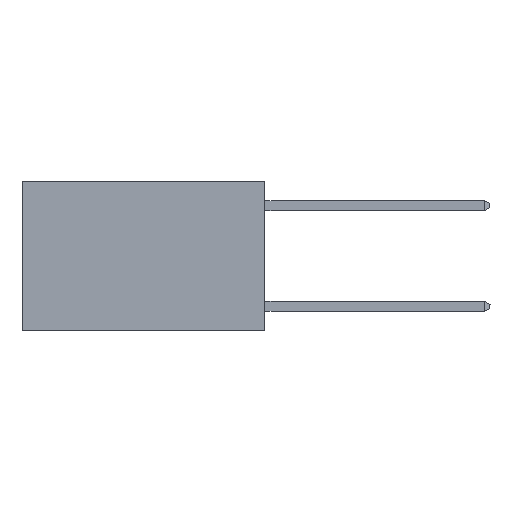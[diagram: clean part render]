
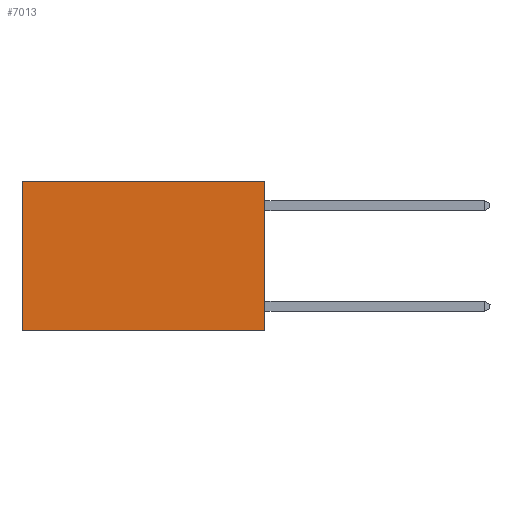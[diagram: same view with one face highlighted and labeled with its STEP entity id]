
A CAD part, left-side view. The second image highlights one B-rep face of the part: STEP entity #7013.
In plain terms, the highlighted planar face has unit normal (-1, 0, 0).
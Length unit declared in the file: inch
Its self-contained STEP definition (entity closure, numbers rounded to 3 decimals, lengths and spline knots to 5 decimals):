
#8 = ORIENTED_EDGE ( 'NONE', *, *, #19755, .T. ) ;
#76 = PLANE ( 'NONE',  #18630 ) ;
#163 = DIRECTION ( 'NONE',  ( 0., 0., -1. ) ) ;
#978 = VECTOR ( 'NONE', #23989, 39.37008 ) ;
#1407 = CARTESIAN_POINT ( 'NONE',  ( 0.2625, 0., -0.37 ) ) ;
#1803 = DIRECTION ( 'NONE',  ( 0., 1., 0. ) ) ;
#2769 = CARTESIAN_POINT ( 'NONE',  ( 0.2625, 0.6, 0. ) ) ;
#3751 = ORIENTED_EDGE ( 'NONE', *, *, #18861, .T. ) ;
#3913 = EDGE_CURVE ( 'NONE', #17899, #15839, #20355, .T. ) ;
#4371 = VERTEX_POINT ( 'NONE', #16931 ) ;
#4446 = DIRECTION ( 'NONE',  ( 0., 0., -1. ) ) ;
#4712 = LINE ( 'NONE', #24178, #14637 ) ;
#6877 = VECTOR ( 'NONE', #10764, 39.37008 ) ;
#7013 = ADVANCED_FACE ( 'NONE', ( #7823 ), #76, .F. ) ;
#7823 = FACE_OUTER_BOUND ( 'NONE', #11026, .T. ) ;
#7838 = EDGE_CURVE ( 'NONE', #10480, #17899, #4712, .T. ) ;
#8039 = CARTESIAN_POINT ( 'NONE',  ( 0.2625, 0., 0. ) ) ;
#9858 = VECTOR ( 'NONE', #1803, 39.37008 ) ;
#10480 = VERTEX_POINT ( 'NONE', #13433 ) ;
#10764 = DIRECTION ( 'NONE',  ( 0., 0., -1. ) ) ;
#11026 = EDGE_LOOP ( 'NONE', ( #8, #15494, #16823, #3751 ) ) ;
#11566 = LINE ( 'NONE', #12212, #978 ) ;
#12099 = DIRECTION ( 'NONE',  ( 1., 0., 0. ) ) ;
#12212 = CARTESIAN_POINT ( 'NONE',  ( 0.2625, 0., 0. ) ) ;
#13433 = CARTESIAN_POINT ( 'NONE',  ( 0.2625, 0., 0. ) ) ;
#14637 = VECTOR ( 'NONE', #4446, 39.37008 ) ;
#15494 = ORIENTED_EDGE ( 'NONE', *, *, #3913, .F. ) ;
#15839 = VERTEX_POINT ( 'NONE', #24863 ) ;
#16823 = ORIENTED_EDGE ( 'NONE', *, *, #7838, .F. ) ;
#16931 = CARTESIAN_POINT ( 'NONE',  ( 0.2625, 0.6, 0. ) ) ;
#17651 = CARTESIAN_POINT ( 'NONE',  ( 0.2625, 0., -0.37 ) ) ;
#17899 = VERTEX_POINT ( 'NONE', #1407 ) ;
#18630 = AXIS2_PLACEMENT_3D ( 'NONE', #8039, #12099, #163 ) ;
#18861 = EDGE_CURVE ( 'NONE', #10480, #4371, #11566, .T. ) ;
#19755 = EDGE_CURVE ( 'NONE', #4371, #15839, #21981, .T. ) ;
#20355 = LINE ( 'NONE', #17651, #9858 ) ;
#21981 = LINE ( 'NONE', #2769, #6877 ) ;
#23989 = DIRECTION ( 'NONE',  ( 0., 1., 0. ) ) ;
#24178 = CARTESIAN_POINT ( 'NONE',  ( 0.2625, 0., 0. ) ) ;
#24863 = CARTESIAN_POINT ( 'NONE',  ( 0.2625, 0.6, -0.37 ) ) ;
